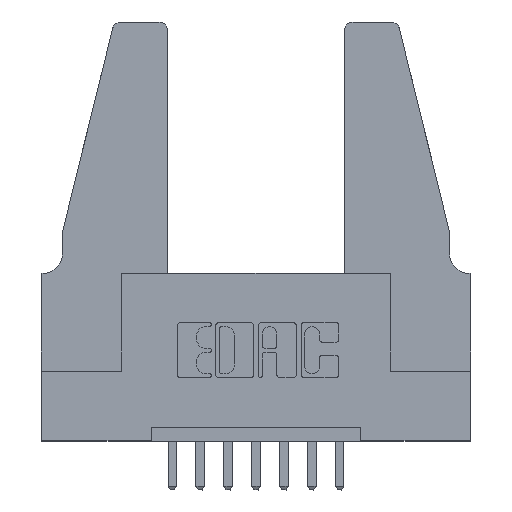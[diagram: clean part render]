
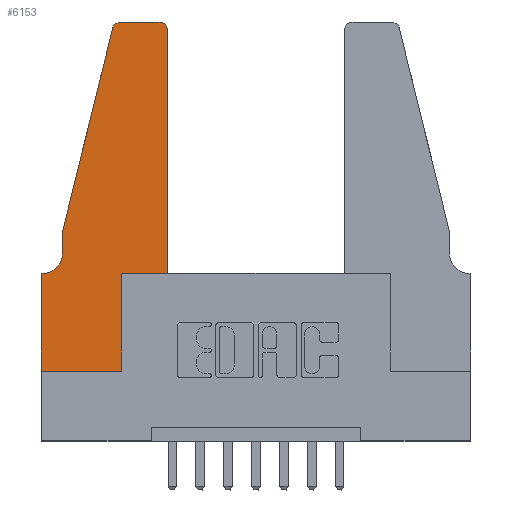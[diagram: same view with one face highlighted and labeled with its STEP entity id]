
A CAD part, top view. The second image highlights one B-rep face of the part: STEP entity #6153.
In plain terms, the highlighted planar face has unit normal (0, 0, 1).
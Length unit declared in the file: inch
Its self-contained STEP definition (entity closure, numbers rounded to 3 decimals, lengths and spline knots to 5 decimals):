
#34 = CARTESIAN_POINT ( 'NONE',  ( 0.0755, 0.5, 0.37 ) ) ;
#72 = CARTESIAN_POINT ( 'NONE',  ( 0.4205, 1.25, 0.37 ) ) ;
#272 = EDGE_CURVE ( 'NONE', #4042, #1567, #5184, .T. ) ;
#307 = DIRECTION ( 'NONE',  ( 1., 0., 0. ) ) ;
#364 = CARTESIAN_POINT ( 'NONE',  ( 0.2865, 0.35, 0.37 ) ) ;
#398 = VECTOR ( 'NONE', #3946, 39.37008 ) ;
#659 = VERTEX_POINT ( 'NONE', #11774 ) ;
#679 = FACE_OUTER_BOUND ( 'NONE', #8571, .T. ) ;
#730 = DIRECTION ( 'NONE',  ( 1., 0., 0. ) ) ;
#813 = ORIENTED_EDGE ( 'NONE', *, *, #11747, .T. ) ;
#873 = VECTOR ( 'NONE', #730, 39.37008 ) ;
#908 = DIRECTION ( 'NONE',  ( 0., -1., 0. ) ) ;
#1119 = LINE ( 'NONE', #3377, #6164 ) ;
#1143 = VECTOR ( 'NONE', #10866, 39.37008 ) ;
#1148 = DIRECTION ( 'NONE',  ( 1., 0., 0. ) ) ;
#1237 = CARTESIAN_POINT ( 'NONE',  ( 0.4505, 1.22, 0.37 ) ) ;
#1254 = DIRECTION ( 'NONE',  ( 0., 0., 1. ) ) ;
#1567 = VERTEX_POINT ( 'NONE', #8190 ) ;
#1604 = DIRECTION ( 'NONE',  ( 0., -1., 0. ) ) ;
#1650 = CARTESIAN_POINT ( 'NONE',  ( 0.4505, 0.35, 0.37 ) ) ;
#1695 = VECTOR ( 'NONE', #3833, 39.37008 ) ;
#1894 = DIRECTION ( 'NONE',  ( -1., 0., 0. ) ) ;
#1979 = AXIS2_PLACEMENT_3D ( 'NONE', #5997, #6799, #1148 ) ;
#2057 = CARTESIAN_POINT ( 'NONE',  ( 0., 0., 0.37 ) ) ;
#2304 = EDGE_CURVE ( 'NONE', #6498, #4042, #4712, .T. ) ;
#2870 = LINE ( 'NONE', #12010, #7423 ) ;
#2929 = VERTEX_POINT ( 'NONE', #3563 ) ;
#3195 = CARTESIAN_POINT ( 'NONE',  ( 0.2865, 0.35, 0.37 ) ) ;
#3275 = PLANE ( 'NONE',  #3630 ) ;
#3364 = EDGE_CURVE ( 'NONE', #9127, #659, #10665, .T. ) ;
#3377 = CARTESIAN_POINT ( 'NONE',  ( 0.0755, 0.35, 0.37 ) ) ;
#3460 = CARTESIAN_POINT ( 'NONE',  ( 0.2865, 0., 0.37 ) ) ;
#3563 = CARTESIAN_POINT ( 'NONE',  ( 0.4505, 0.35, 0.37 ) ) ;
#3630 = AXIS2_PLACEMENT_3D ( 'NONE', #4339, #9880, #9925 ) ;
#3703 = ORIENTED_EDGE ( 'NONE', *, *, #6666, .T. ) ;
#3730 = CARTESIAN_POINT ( 'NONE',  ( 0.284, 1.25, 0.37 ) ) ;
#3833 = DIRECTION ( 'NONE',  ( 0., 1., 0. ) ) ;
#3946 = DIRECTION ( 'NONE',  ( 1., 0., 0. ) ) ;
#4042 = VERTEX_POINT ( 'NONE', #4819 ) ;
#4212 = LINE ( 'NONE', #6712, #1695 ) ;
#4219 = CARTESIAN_POINT ( 'NONE',  ( 0., 0., 0.37 ) ) ;
#4339 = CARTESIAN_POINT ( 'NONE',  ( 0., 0.35, 0.37 ) ) ;
#4437 = EDGE_CURVE ( 'NONE', #9827, #9127, #12052, .T. ) ;
#4712 = LINE ( 'NONE', #34, #10168 ) ;
#4819 = CARTESIAN_POINT ( 'NONE',  ( 0.0755, 0.42, 0.37 ) ) ;
#4824 = DIRECTION ( 'NONE',  ( 0., 0., -1. ) ) ;
#4943 = ORIENTED_EDGE ( 'NONE', *, *, #10077, .T. ) ;
#4944 = VECTOR ( 'NONE', #6930, 39.37008 ) ;
#5002 = EDGE_CURVE ( 'NONE', #2929, #12166, #4212, .T. ) ;
#5162 = AXIS2_PLACEMENT_3D ( 'NONE', #9478, #4824, #1894 ) ;
#5184 = CIRCLE ( 'NONE', #5162, 0.07 ) ;
#5856 = EDGE_CURVE ( 'NONE', #6710, #12162, #2870, .T. ) ;
#5932 = ORIENTED_EDGE ( 'NONE', *, *, #2304, .T. ) ;
#5997 = CARTESIAN_POINT ( 'NONE',  ( 0.4205, 1.22, 0.37 ) ) ;
#6153 = ADVANCED_FACE ( 'NONE', ( #679 ), #3275, .T. ) ;
#6164 = VECTOR ( 'NONE', #8000, 39.37008 ) ;
#6237 = CARTESIAN_POINT ( 'NONE',  ( 0.0755, 0.5, 0.37 ) ) ;
#6288 = EDGE_CURVE ( 'NONE', #12166, #9827, #9723, .T. ) ;
#6337 = EDGE_CURVE ( 'NONE', #659, #6498, #11200, .T. ) ;
#6498 = VERTEX_POINT ( 'NONE', #9632 ) ;
#6666 = EDGE_CURVE ( 'NONE', #7941, #6920, #12187, .T. ) ;
#6710 = VERTEX_POINT ( 'NONE', #7769 ) ;
#6712 = CARTESIAN_POINT ( 'NONE',  ( 0.4505, 0.35, 0.37 ) ) ;
#6799 = DIRECTION ( 'NONE',  ( 0., 0., 1. ) ) ;
#6876 = VECTOR ( 'NONE', #9155, 39.37008 ) ;
#6920 = VERTEX_POINT ( 'NONE', #3195 ) ;
#6930 = DIRECTION ( 'NONE',  ( 0., 1., 0. ) ) ;
#7239 = AXIS2_PLACEMENT_3D ( 'NONE', #11634, #1254, #307 ) ;
#7423 = VECTOR ( 'NONE', #1604, 39.37008 ) ;
#7769 = CARTESIAN_POINT ( 'NONE',  ( 0., 0.35, 0.37 ) ) ;
#7941 = VERTEX_POINT ( 'NONE', #3460 ) ;
#8000 = DIRECTION ( 'NONE',  ( -1., 0., 0. ) ) ;
#8122 = LINE ( 'NONE', #1650, #873 ) ;
#8190 = CARTESIAN_POINT ( 'NONE',  ( 0.0055, 0.35, 0.37 ) ) ;
#8213 = ORIENTED_EDGE ( 'NONE', *, *, #5002, .T. ) ;
#8571 = EDGE_LOOP ( 'NONE', ( #9260, #11624, #8848, #5932, #11812, #813, #12015, #9246, #3703, #4943, #8213, #9566 ) ) ;
#8848 = ORIENTED_EDGE ( 'NONE', *, *, #6337, .T. ) ;
#9127 = VERTEX_POINT ( 'NONE', #3730 ) ;
#9155 = DIRECTION ( 'NONE',  ( -1., 0., 0. ) ) ;
#9246 = ORIENTED_EDGE ( 'NONE', *, *, #11416, .T. ) ;
#9260 = ORIENTED_EDGE ( 'NONE', *, *, #4437, .T. ) ;
#9478 = CARTESIAN_POINT ( 'NONE',  ( 0.0055, 0.42, 0.37 ) ) ;
#9566 = ORIENTED_EDGE ( 'NONE', *, *, #6288, .T. ) ;
#9632 = CARTESIAN_POINT ( 'NONE',  ( 0.0755, 0.5, 0.37 ) ) ;
#9723 = CIRCLE ( 'NONE', #1979, 0.03 ) ;
#9827 = VERTEX_POINT ( 'NONE', #72 ) ;
#9880 = DIRECTION ( 'NONE',  ( 0., 0., 1. ) ) ;
#9925 = DIRECTION ( 'NONE',  ( 1., 0., 0. ) ) ;
#10077 = EDGE_CURVE ( 'NONE', #6920, #2929, #8122, .T. ) ;
#10168 = VECTOR ( 'NONE', #908, 39.37008 ) ;
#10665 = CIRCLE ( 'NONE', #7239, 0.03 ) ;
#10866 = DIRECTION ( 'NONE',  ( -0.239, -0.971, 0. ) ) ;
#11200 = LINE ( 'NONE', #6237, #1143 ) ;
#11416 = EDGE_CURVE ( 'NONE', #12162, #7941, #11488, .T. ) ;
#11488 = LINE ( 'NONE', #2057, #398 ) ;
#11624 = ORIENTED_EDGE ( 'NONE', *, *, #3364, .T. ) ;
#11634 = CARTESIAN_POINT ( 'NONE',  ( 0.284, 1.22, 0.37 ) ) ;
#11747 = EDGE_CURVE ( 'NONE', #1567, #6710, #1119, .T. ) ;
#11774 = CARTESIAN_POINT ( 'NONE',  ( 0.25487, 1.22718, 0.37 ) ) ;
#11812 = ORIENTED_EDGE ( 'NONE', *, *, #272, .T. ) ;
#11969 = CARTESIAN_POINT ( 'NONE',  ( 0.2605, 1.25, 0.37 ) ) ;
#12010 = CARTESIAN_POINT ( 'NONE',  ( 0., 0., 0.37 ) ) ;
#12015 = ORIENTED_EDGE ( 'NONE', *, *, #5856, .T. ) ;
#12052 = LINE ( 'NONE', #11969, #6876 ) ;
#12162 = VERTEX_POINT ( 'NONE', #4219 ) ;
#12166 = VERTEX_POINT ( 'NONE', #1237 ) ;
#12187 = LINE ( 'NONE', #364, #4944 ) ;
